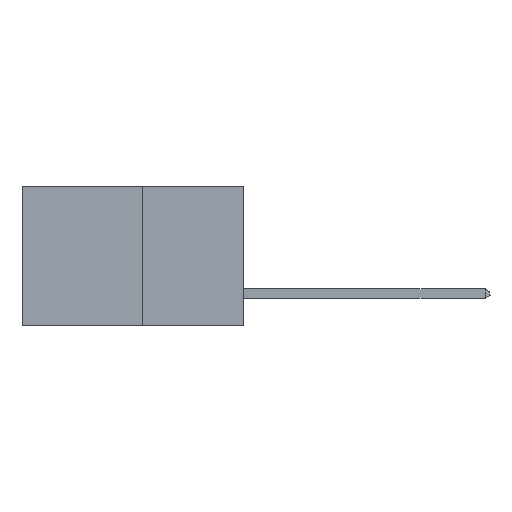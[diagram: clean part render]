
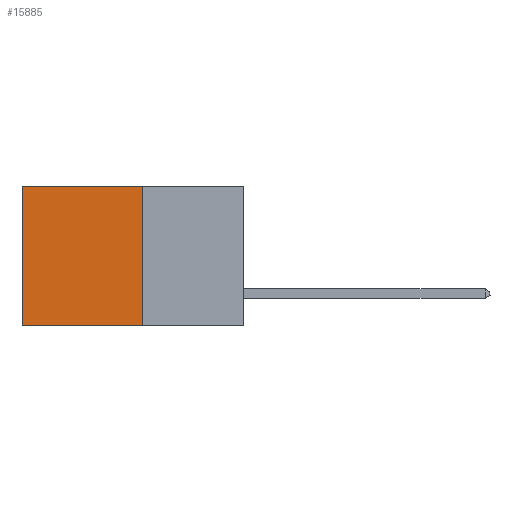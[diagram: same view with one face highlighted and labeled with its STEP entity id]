
A CAD part, left-side view. The second image highlights one B-rep face of the part: STEP entity #15885.
In plain terms, the highlighted planar face has unit normal (-1, 0, 0).
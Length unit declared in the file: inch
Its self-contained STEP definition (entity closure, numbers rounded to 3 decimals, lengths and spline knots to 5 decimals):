
#184 = LINE ( 'NONE', #24760, #15297 ) ;
#1936 = PLANE ( 'NONE',  #12897 ) ;
#3644 = CARTESIAN_POINT ( 'NONE',  ( 0.277, 0.27, -0.37 ) ) ;
#5641 = DIRECTION ( 'NONE',  ( 0., 0., -1. ) ) ;
#7001 = EDGE_LOOP ( 'NONE', ( #11412, #17813, #13934, #13973 ) ) ;
#7825 = EDGE_CURVE ( 'NONE', #13957, #8108, #184, .T. ) ;
#8108 = VERTEX_POINT ( 'NONE', #8158 ) ;
#8158 = CARTESIAN_POINT ( 'NONE',  ( 0.277, 0.59, -0.37 ) ) ;
#8229 = CARTESIAN_POINT ( 'NONE',  ( 0.277, 0.27, 0. ) ) ;
#8341 = FACE_OUTER_BOUND ( 'NONE', #7001, .T. ) ;
#8373 = DIRECTION ( 'NONE',  ( 0., 1., 0. ) ) ;
#10806 = CARTESIAN_POINT ( 'NONE',  ( 0.277, 0.59, 0. ) ) ;
#11412 = ORIENTED_EDGE ( 'NONE', *, *, #7825, .T. ) ;
#11846 = CARTESIAN_POINT ( 'NONE',  ( 0.277, 0.27, -0.37 ) ) ;
#12897 = AXIS2_PLACEMENT_3D ( 'NONE', #11846, #22424, #13804 ) ;
#13804 = DIRECTION ( 'NONE',  ( 0., 0., -1. ) ) ;
#13881 = CARTESIAN_POINT ( 'NONE',  ( 0.277, 0.27, -0.37 ) ) ;
#13934 = ORIENTED_EDGE ( 'NONE', *, *, #14192, .F. ) ;
#13957 = VERTEX_POINT ( 'NONE', #10806 ) ;
#13973 = ORIENTED_EDGE ( 'NONE', *, *, #14678, .T. ) ;
#14192 = EDGE_CURVE ( 'NONE', #21094, #21008, #14502, .T. ) ;
#14502 = LINE ( 'NONE', #3644, #24195 ) ;
#14678 = EDGE_CURVE ( 'NONE', #21094, #13957, #18201, .T. ) ;
#14825 = VECTOR ( 'NONE', #15835, 39.37008 ) ;
#15161 = DIRECTION ( 'NONE',  ( 0., 0., -1. ) ) ;
#15297 = VECTOR ( 'NONE', #15161, 39.37008 ) ;
#15749 = CARTESIAN_POINT ( 'NONE',  ( 0.277, 0.27, -0.37 ) ) ;
#15835 = DIRECTION ( 'NONE',  ( 0., 1., 0. ) ) ;
#15885 = ADVANCED_FACE ( 'NONE', ( #8341 ), #1936, .F. ) ;
#17605 = VECTOR ( 'NONE', #8373, 39.37008 ) ;
#17813 = ORIENTED_EDGE ( 'NONE', *, *, #21020, .F. ) ;
#18201 = LINE ( 'NONE', #18691, #17605 ) ;
#18691 = CARTESIAN_POINT ( 'NONE',  ( 0.277, 0.27, 0. ) ) ;
#21008 = VERTEX_POINT ( 'NONE', #15749 ) ;
#21020 = EDGE_CURVE ( 'NONE', #21008, #8108, #25070, .T. ) ;
#21094 = VERTEX_POINT ( 'NONE', #8229 ) ;
#22424 = DIRECTION ( 'NONE',  ( 1., 0., 0. ) ) ;
#24195 = VECTOR ( 'NONE', #5641, 39.37008 ) ;
#24760 = CARTESIAN_POINT ( 'NONE',  ( 0.277, 0.59, -0.37 ) ) ;
#25070 = LINE ( 'NONE', #13881, #14825 ) ;
